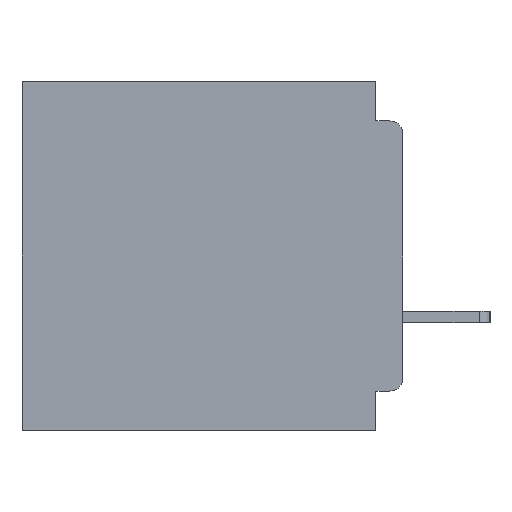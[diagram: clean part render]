
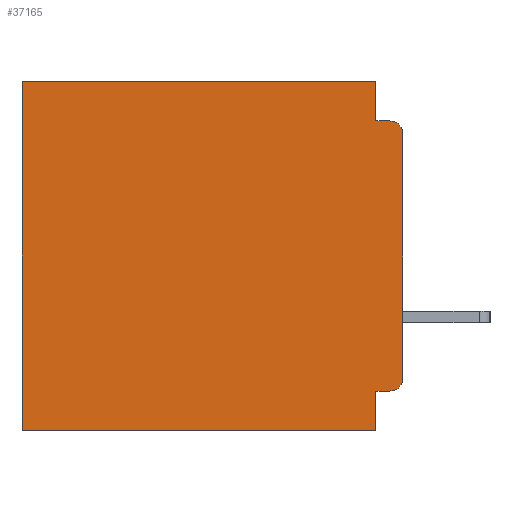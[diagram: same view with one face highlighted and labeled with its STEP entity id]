
A CAD part, left-side view. The second image highlights one B-rep face of the part: STEP entity #37165.
In plain terms, the highlighted planar face has unit normal (-1, 0, 0).
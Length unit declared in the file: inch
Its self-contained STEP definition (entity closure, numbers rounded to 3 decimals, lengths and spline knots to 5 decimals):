
#294 = CARTESIAN_POINT ( 'NONE',  ( 0.3, 0.031, -0.045 ) ) ;
#469 = ORIENTED_EDGE ( 'NONE', *, *, #1948, .F. ) ;
#700 = CARTESIAN_POINT ( 'NONE',  ( 0.3, 0., -0.355 ) ) ;
#712 = CIRCLE ( 'NONE', #16001, 0.015 ) ;
#949 = ORIENTED_EDGE ( 'NONE', *, *, #47294, .F. ) ;
#1066 = CIRCLE ( 'NONE', #13392, 0.015 ) ;
#1238 = DIRECTION ( 'NONE',  ( 0., 0., -1. ) ) ;
#1948 = EDGE_CURVE ( 'NONE', #47673, #23932, #6043, .T. ) ;
#2168 = VECTOR ( 'NONE', #2838, 39.37008 ) ;
#2282 = AXIS2_PLACEMENT_3D ( 'NONE', #49662, #30613, #7260 ) ;
#2838 = DIRECTION ( 'NONE',  ( 0., -1., 0. ) ) ;
#2868 = EDGE_CURVE ( 'NONE', #27754, #28996, #23074, .T. ) ;
#3351 = EDGE_CURVE ( 'NONE', #45191, #10519, #1066, .T. ) ;
#3977 = ORIENTED_EDGE ( 'NONE', *, *, #15842, .F. ) ;
#4634 = DIRECTION ( 'NONE',  ( 0., 1., 0. ) ) ;
#4642 = LINE ( 'NONE', #6730, #2168 ) ;
#5020 = CARTESIAN_POINT ( 'NONE',  ( 0.3, 0.031, -0.355 ) ) ;
#6043 = LINE ( 'NONE', #6265, #25601 ) ;
#6265 = CARTESIAN_POINT ( 'NONE',  ( 0.3, 0.031, -0.4 ) ) ;
#6730 = CARTESIAN_POINT ( 'NONE',  ( 0.3, 0., -0.045 ) ) ;
#7260 = DIRECTION ( 'NONE',  ( 0., 0., -1. ) ) ;
#8379 = CARTESIAN_POINT ( 'NONE',  ( 0.3, 0.437, -0.4 ) ) ;
#8803 = LINE ( 'NONE', #28823, #47665 ) ;
#10062 = CARTESIAN_POINT ( 'NONE',  ( 0.3, 0.437, 0. ) ) ;
#10519 = VERTEX_POINT ( 'NONE', #29766 ) ;
#10887 = CARTESIAN_POINT ( 'NONE',  ( 0.3, 0., -0.06 ) ) ;
#11127 = CARTESIAN_POINT ( 'NONE',  ( 0.3, 0.015, -0.34 ) ) ;
#11181 = CARTESIAN_POINT ( 'NONE',  ( 0.3, 0.015, -0.06 ) ) ;
#12908 = DIRECTION ( 'NONE',  ( 0., 0., -1. ) ) ;
#13246 = ORIENTED_EDGE ( 'NONE', *, *, #31104, .F. ) ;
#13392 = AXIS2_PLACEMENT_3D ( 'NONE', #11127, #38332, #15116 ) ;
#14353 = VERTEX_POINT ( 'NONE', #19165 ) ;
#15000 = ORIENTED_EDGE ( 'NONE', *, *, #20275, .F. ) ;
#15116 = DIRECTION ( 'NONE',  ( 0., 0., -1. ) ) ;
#15164 = DIRECTION ( 'NONE',  ( 0., 0., -1. ) ) ;
#15278 = DIRECTION ( 'NONE',  ( 0., 1., 0. ) ) ;
#15842 = EDGE_CURVE ( 'NONE', #22317, #10519, #15981, .T. ) ;
#15981 = LINE ( 'NONE', #28499, #45644 ) ;
#16001 = AXIS2_PLACEMENT_3D ( 'NONE', #11181, #38378, #15164 ) ;
#19165 = CARTESIAN_POINT ( 'NONE',  ( 0.3, 0.015, -0.045 ) ) ;
#20275 = EDGE_CURVE ( 'NONE', #27754, #45731, #8803, .T. ) ;
#21031 = CARTESIAN_POINT ( 'NONE',  ( 0.3, 0., 0. ) ) ;
#22317 = VERTEX_POINT ( 'NONE', #10887 ) ;
#23074 = LINE ( 'NONE', #21031, #32179 ) ;
#23913 = DIRECTION ( 'NONE',  ( 0., 0., -1. ) ) ;
#23932 = VERTEX_POINT ( 'NONE', #33492 ) ;
#24715 = ORIENTED_EDGE ( 'NONE', *, *, #44953, .T. ) ;
#24803 = ORIENTED_EDGE ( 'NONE', *, *, #46384, .T. ) ;
#25601 = VECTOR ( 'NONE', #12908, 39.37008 ) ;
#25755 = FACE_OUTER_BOUND ( 'NONE', #26922, .T. ) ;
#26556 = PLANE ( 'NONE',  #2282 ) ;
#26922 = EDGE_LOOP ( 'NONE', ( #3977, #24715, #949, #15000, #48305, #24803, #30313, #469, #13246, #37585 ) ) ;
#27754 = VERTEX_POINT ( 'NONE', #37356 ) ;
#27811 = CARTESIAN_POINT ( 'NONE',  ( 0.3, 0.437, -0.4 ) ) ;
#28227 = CARTESIAN_POINT ( 'NONE',  ( 0.3, 0.015, -0.355 ) ) ;
#28499 = CARTESIAN_POINT ( 'NONE',  ( 0.3, 0., -0.4 ) ) ;
#28823 = CARTESIAN_POINT ( 'NONE',  ( 0.3, 0.031, 0. ) ) ;
#28899 = CARTESIAN_POINT ( 'NONE',  ( 0.3, 0., -0.4 ) ) ;
#28996 = VERTEX_POINT ( 'NONE', #10062 ) ;
#29766 = CARTESIAN_POINT ( 'NONE',  ( 0.3, 0., -0.34 ) ) ;
#30313 = ORIENTED_EDGE ( 'NONE', *, *, #31363, .F. ) ;
#30613 = DIRECTION ( 'NONE',  ( 1., 0., 0. ) ) ;
#31104 = EDGE_CURVE ( 'NONE', #45191, #47673, #36627, .T. ) ;
#31363 = EDGE_CURVE ( 'NONE', #23932, #49485, #33594, .T. ) ;
#32179 = VECTOR ( 'NONE', #15278, 39.37008 ) ;
#32714 = DIRECTION ( 'NONE',  ( 0., 0., -1. ) ) ;
#32783 = DIRECTION ( 'NONE',  ( 0., 1., 0. ) ) ;
#33492 = CARTESIAN_POINT ( 'NONE',  ( 0.3, 0.031, -0.4 ) ) ;
#33594 = LINE ( 'NONE', #28899, #34820 ) ;
#34820 = VECTOR ( 'NONE', #32783, 39.37008 ) ;
#35765 = VECTOR ( 'NONE', #23913, 39.37008 ) ;
#36627 = LINE ( 'NONE', #700, #45661 ) ;
#37165 = ADVANCED_FACE ( 'NONE', ( #25755 ), #26556, .F. ) ;
#37356 = CARTESIAN_POINT ( 'NONE',  ( 0.3, 0.031, 0. ) ) ;
#37585 = ORIENTED_EDGE ( 'NONE', *, *, #3351, .T. ) ;
#38332 = DIRECTION ( 'NONE',  ( -1., 0., 0. ) ) ;
#38378 = DIRECTION ( 'NONE',  ( -1., 0., 0. ) ) ;
#44953 = EDGE_CURVE ( 'NONE', #22317, #14353, #712, .T. ) ;
#45191 = VERTEX_POINT ( 'NONE', #28227 ) ;
#45644 = VECTOR ( 'NONE', #1238, 39.37008 ) ;
#45661 = VECTOR ( 'NONE', #4634, 39.37008 ) ;
#45731 = VERTEX_POINT ( 'NONE', #294 ) ;
#45997 = LINE ( 'NONE', #27811, #35765 ) ;
#46384 = EDGE_CURVE ( 'NONE', #28996, #49485, #45997, .T. ) ;
#47294 = EDGE_CURVE ( 'NONE', #45731, #14353, #4642, .T. ) ;
#47665 = VECTOR ( 'NONE', #32714, 39.37008 ) ;
#47673 = VERTEX_POINT ( 'NONE', #5020 ) ;
#48305 = ORIENTED_EDGE ( 'NONE', *, *, #2868, .T. ) ;
#49485 = VERTEX_POINT ( 'NONE', #8379 ) ;
#49662 = CARTESIAN_POINT ( 'NONE',  ( 0.3, 0., -0.4 ) ) ;
